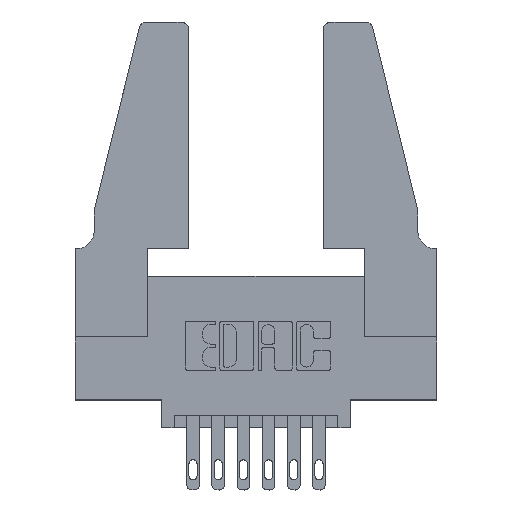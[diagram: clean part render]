
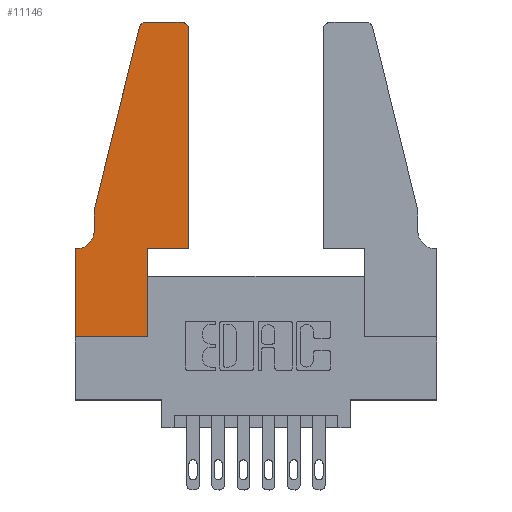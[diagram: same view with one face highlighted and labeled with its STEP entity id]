
A CAD part, top view. The second image highlights one B-rep face of the part: STEP entity #11146.
In plain terms, the highlighted planar face has unit normal (0, 0, 1).
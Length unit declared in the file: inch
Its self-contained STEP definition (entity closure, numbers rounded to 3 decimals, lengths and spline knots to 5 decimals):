
#171 = ORIENTED_EDGE ( 'NONE', *, *, #9764, .T. ) ;
#291 = CARTESIAN_POINT ( 'NONE',  ( 0., 0., 0.37 ) ) ;
#343 = VERTEX_POINT ( 'NONE', #1500 ) ;
#513 = EDGE_CURVE ( 'NONE', #343, #11352, #11130, .T. ) ;
#635 = ORIENTED_EDGE ( 'NONE', *, *, #4137, .T. ) ;
#675 = ORIENTED_EDGE ( 'NONE', *, *, #11398, .T. ) ;
#740 = CARTESIAN_POINT ( 'NONE',  ( 0.4505, 0.35, 0.37 ) ) ;
#761 = DIRECTION ( 'NONE',  ( 0., 0., 1. ) ) ;
#830 = CARTESIAN_POINT ( 'NONE',  ( 0.0755, 0.5, 0.37 ) ) ;
#847 = LINE ( 'NONE', #740, #7291 ) ;
#1156 = AXIS2_PLACEMENT_3D ( 'NONE', #7612, #9562, #5906 ) ;
#1207 = EDGE_CURVE ( 'NONE', #4948, #7060, #6725, .T. ) ;
#1331 = LINE ( 'NONE', #9942, #8303 ) ;
#1500 = CARTESIAN_POINT ( 'NONE',  ( 0.0755, 0.42, 0.37 ) ) ;
#1675 = DIRECTION ( 'NONE',  ( 1., 0., 0. ) ) ;
#1851 = DIRECTION ( 'NONE',  ( 0., -1., 0. ) ) ;
#1953 = DIRECTION ( 'NONE',  ( 0., 0., -1. ) ) ;
#2092 = EDGE_CURVE ( 'NONE', #7877, #4090, #2853, .T. ) ;
#2204 = CARTESIAN_POINT ( 'NONE',  ( 0.0755, 0.5, 0.37 ) ) ;
#2336 = CARTESIAN_POINT ( 'NONE',  ( 0.2865, 0.35, 0.37 ) ) ;
#2477 = VECTOR ( 'NONE', #10148, 39.37008 ) ;
#2580 = ORIENTED_EDGE ( 'NONE', *, *, #5733, .T. ) ;
#2853 = CIRCLE ( 'NONE', #8324, 0.03 ) ;
#2863 = DIRECTION ( 'NONE',  ( 1., 0., 0. ) ) ;
#2978 = DIRECTION ( 'NONE',  ( -1., 0., 0. ) ) ;
#2993 = LINE ( 'NONE', #9086, #4725 ) ;
#3427 = CARTESIAN_POINT ( 'NONE',  ( 0., 0.35, 0.37 ) ) ;
#3446 = ORIENTED_EDGE ( 'NONE', *, *, #2092, .T. ) ;
#3673 = DIRECTION ( 'NONE',  ( -0.239, -0.971, 0. ) ) ;
#3677 = VERTEX_POINT ( 'NONE', #2204 ) ;
#3814 = LINE ( 'NONE', #830, #10772 ) ;
#4090 = VERTEX_POINT ( 'NONE', #6173 ) ;
#4137 = EDGE_CURVE ( 'NONE', #7060, #3677, #3814, .T. ) ;
#4339 = ORIENTED_EDGE ( 'NONE', *, *, #9656, .T. ) ;
#4359 = EDGE_LOOP ( 'NONE', ( #6560, #7971, #635, #4339, #9331, #9070, #8585, #2580, #675, #171, #8425, #3446 ) ) ;
#4531 = CARTESIAN_POINT ( 'NONE',  ( 0.25487, 1.22718, 0.37 ) ) ;
#4548 = DIRECTION ( 'NONE',  ( 1., 0., 0. ) ) ;
#4558 = VERTEX_POINT ( 'NONE', #291 ) ;
#4587 = CARTESIAN_POINT ( 'NONE',  ( 0.2605, 1.25, 0.37 ) ) ;
#4720 = EDGE_CURVE ( 'NONE', #7550, #7877, #7629, .T. ) ;
#4725 = VECTOR ( 'NONE', #1851, 39.37008 ) ;
#4948 = VERTEX_POINT ( 'NONE', #10319 ) ;
#5052 = EDGE_CURVE ( 'NONE', #10874, #4558, #1331, .T. ) ;
#5065 = AXIS2_PLACEMENT_3D ( 'NONE', #5706, #1953, #7461 ) ;
#5161 = CARTESIAN_POINT ( 'NONE',  ( 0.284, 1.22, 0.37 ) ) ;
#5231 = EDGE_CURVE ( 'NONE', #4090, #4948, #5505, .T. ) ;
#5505 = LINE ( 'NONE', #4587, #2477 ) ;
#5702 = CARTESIAN_POINT ( 'NONE',  ( 0., 0., 0.37 ) ) ;
#5706 = CARTESIAN_POINT ( 'NONE',  ( 0.0055, 0.42, 0.37 ) ) ;
#5733 = EDGE_CURVE ( 'NONE', #4558, #6888, #9038, .T. ) ;
#5792 = VECTOR ( 'NONE', #10474, 39.37008 ) ;
#5906 = DIRECTION ( 'NONE',  ( 1., 0., 0. ) ) ;
#5986 = CARTESIAN_POINT ( 'NONE',  ( 0.4505, 0.35, 0.37 ) ) ;
#6069 = EDGE_CURVE ( 'NONE', #11352, #10874, #6375, .T. ) ;
#6114 = DIRECTION ( 'NONE',  ( 0., 0., 1. ) ) ;
#6173 = CARTESIAN_POINT ( 'NONE',  ( 0.4205, 1.25, 0.37 ) ) ;
#6375 = LINE ( 'NONE', #8397, #11179 ) ;
#6540 = VECTOR ( 'NONE', #6942, 39.37008 ) ;
#6560 = ORIENTED_EDGE ( 'NONE', *, *, #5231, .T. ) ;
#6605 = AXIS2_PLACEMENT_3D ( 'NONE', #5161, #6114, #7923 ) ;
#6674 = FACE_OUTER_BOUND ( 'NONE', #4359, .T. ) ;
#6725 = CIRCLE ( 'NONE', #6605, 0.03 ) ;
#6888 = VERTEX_POINT ( 'NONE', #7155 ) ;
#6942 = DIRECTION ( 'NONE',  ( 0., 1., 0. ) ) ;
#7060 = VERTEX_POINT ( 'NONE', #4531 ) ;
#7155 = CARTESIAN_POINT ( 'NONE',  ( 0.2865, 0., 0.37 ) ) ;
#7291 = VECTOR ( 'NONE', #4548, 39.37008 ) ;
#7461 = DIRECTION ( 'NONE',  ( -1., 0., 0. ) ) ;
#7550 = VERTEX_POINT ( 'NONE', #10908 ) ;
#7612 = CARTESIAN_POINT ( 'NONE',  ( 0., 0.35, 0.37 ) ) ;
#7629 = LINE ( 'NONE', #5986, #5792 ) ;
#7877 = VERTEX_POINT ( 'NONE', #10468 ) ;
#7923 = DIRECTION ( 'NONE',  ( 1., 0., 0. ) ) ;
#7938 = VERTEX_POINT ( 'NONE', #2336 ) ;
#7971 = ORIENTED_EDGE ( 'NONE', *, *, #1207, .T. ) ;
#8063 = LINE ( 'NONE', #11437, #6540 ) ;
#8303 = VECTOR ( 'NONE', #8923, 39.37008 ) ;
#8324 = AXIS2_PLACEMENT_3D ( 'NONE', #10762, #761, #1675 ) ;
#8397 = CARTESIAN_POINT ( 'NONE',  ( 0.0755, 0.35, 0.37 ) ) ;
#8425 = ORIENTED_EDGE ( 'NONE', *, *, #4720, .T. ) ;
#8585 = ORIENTED_EDGE ( 'NONE', *, *, #5052, .T. ) ;
#8923 = DIRECTION ( 'NONE',  ( 0., -1., 0. ) ) ;
#9038 = LINE ( 'NONE', #5702, #11748 ) ;
#9070 = ORIENTED_EDGE ( 'NONE', *, *, #6069, .T. ) ;
#9086 = CARTESIAN_POINT ( 'NONE',  ( 0.0755, 0.5, 0.37 ) ) ;
#9331 = ORIENTED_EDGE ( 'NONE', *, *, #513, .T. ) ;
#9562 = DIRECTION ( 'NONE',  ( 0., 0., 1. ) ) ;
#9656 = EDGE_CURVE ( 'NONE', #3677, #343, #2993, .T. ) ;
#9710 = CARTESIAN_POINT ( 'NONE',  ( 0.0055, 0.35, 0.37 ) ) ;
#9764 = EDGE_CURVE ( 'NONE', #7938, #7550, #847, .T. ) ;
#9942 = CARTESIAN_POINT ( 'NONE',  ( 0., 0., 0.37 ) ) ;
#10148 = DIRECTION ( 'NONE',  ( -1., 0., 0. ) ) ;
#10319 = CARTESIAN_POINT ( 'NONE',  ( 0.284, 1.25, 0.37 ) ) ;
#10468 = CARTESIAN_POINT ( 'NONE',  ( 0.4505, 1.22, 0.37 ) ) ;
#10474 = DIRECTION ( 'NONE',  ( 0., 1., 0. ) ) ;
#10762 = CARTESIAN_POINT ( 'NONE',  ( 0.4205, 1.22, 0.37 ) ) ;
#10772 = VECTOR ( 'NONE', #3673, 39.37008 ) ;
#10874 = VERTEX_POINT ( 'NONE', #3427 ) ;
#10908 = CARTESIAN_POINT ( 'NONE',  ( 0.4505, 0.35, 0.37 ) ) ;
#11130 = CIRCLE ( 'NONE', #5065, 0.07 ) ;
#11146 = ADVANCED_FACE ( 'NONE', ( #6674 ), #11170, .T. ) ;
#11170 = PLANE ( 'NONE',  #1156 ) ;
#11179 = VECTOR ( 'NONE', #2978, 39.37008 ) ;
#11352 = VERTEX_POINT ( 'NONE', #9710 ) ;
#11398 = EDGE_CURVE ( 'NONE', #6888, #7938, #8063, .T. ) ;
#11437 = CARTESIAN_POINT ( 'NONE',  ( 0.2865, 0.35, 0.37 ) ) ;
#11748 = VECTOR ( 'NONE', #2863, 39.37008 ) ;
